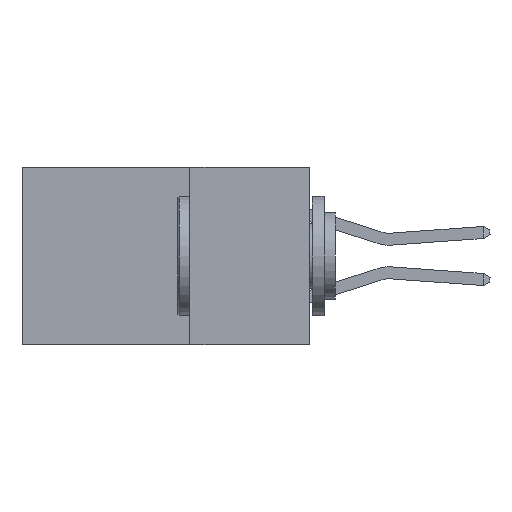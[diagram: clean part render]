
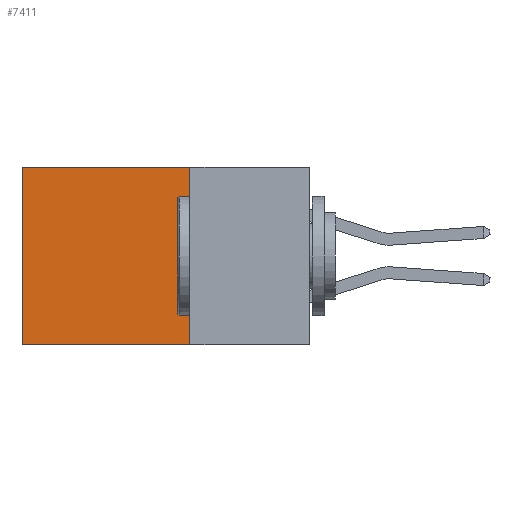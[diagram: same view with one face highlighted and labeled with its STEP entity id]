
A CAD part, left-side view. The second image highlights one B-rep face of the part: STEP entity #7411.
In plain terms, the highlighted planar face has unit normal (-1, 0, 0).
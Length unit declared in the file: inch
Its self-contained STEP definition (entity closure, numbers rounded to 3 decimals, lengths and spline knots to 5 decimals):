
#46 = CARTESIAN_POINT ( 'NONE',  ( 0.298, 0.6, -0.37 ) ) ;
#125 = VECTOR ( 'NONE', #10347, 39.37008 ) ;
#994 = CARTESIAN_POINT ( 'NONE',  ( 0.298, 0.25, 0. ) ) ;
#2013 = DIRECTION ( 'NONE',  ( 0., 1., 0. ) ) ;
#2755 = ORIENTED_EDGE ( 'NONE', *, *, #14834, .T. ) ;
#2896 = DIRECTION ( 'NONE',  ( 1., 0., 0. ) ) ;
#3699 = CARTESIAN_POINT ( 'NONE',  ( 0.298, 0.25, 0. ) ) ;
#4973 = ORIENTED_EDGE ( 'NONE', *, *, #9834, .F. ) ;
#5698 = VECTOR ( 'NONE', #7723, 39.37008 ) ;
#7411 = ADVANCED_FACE ( 'NONE', ( #11401 ), #12450, .F. ) ;
#7413 = ORIENTED_EDGE ( 'NONE', *, *, #21066, .T. ) ;
#7723 = DIRECTION ( 'NONE',  ( 0., 0., -1. ) ) ;
#9039 = EDGE_LOOP ( 'NONE', ( #2755, #11001, #4973, #7413 ) ) ;
#9103 = CARTESIAN_POINT ( 'NONE',  ( 0.298, 0.25, -0.37 ) ) ;
#9834 = EDGE_CURVE ( 'NONE', #15513, #27654, #18242, .T. ) ;
#10347 = DIRECTION ( 'NONE',  ( 0., 1., 0. ) ) ;
#11001 = ORIENTED_EDGE ( 'NONE', *, *, #12710, .F. ) ;
#11401 = FACE_OUTER_BOUND ( 'NONE', #9039, .T. ) ;
#12450 = PLANE ( 'NONE',  #20560 ) ;
#12710 = EDGE_CURVE ( 'NONE', #27654, #29159, #29627, .T. ) ;
#13726 = VERTEX_POINT ( 'NONE', #20423 ) ;
#14834 = EDGE_CURVE ( 'NONE', #13726, #29159, #23051, .T. ) ;
#15513 = VERTEX_POINT ( 'NONE', #3699 ) ;
#16161 = DIRECTION ( 'NONE',  ( 0., 0., -1. ) ) ;
#16728 = VECTOR ( 'NONE', #16161, 39.37008 ) ;
#18242 = LINE ( 'NONE', #21775, #5698 ) ;
#18309 = CARTESIAN_POINT ( 'NONE',  ( 0.298, 0.6, 0. ) ) ;
#19152 = CARTESIAN_POINT ( 'NONE',  ( 0.298, 0.25, 0. ) ) ;
#19452 = DIRECTION ( 'NONE',  ( 0., 0., -1. ) ) ;
#20139 = LINE ( 'NONE', #994, #125 ) ;
#20423 = CARTESIAN_POINT ( 'NONE',  ( 0.298, 0.6, 0. ) ) ;
#20560 = AXIS2_PLACEMENT_3D ( 'NONE', #19152, #2896, #19452 ) ;
#20646 = CARTESIAN_POINT ( 'NONE',  ( 0.298, 0.25, -0.37 ) ) ;
#21066 = EDGE_CURVE ( 'NONE', #15513, #13726, #20139, .T. ) ;
#21775 = CARTESIAN_POINT ( 'NONE',  ( 0.298, 0.25, 0. ) ) ;
#23051 = LINE ( 'NONE', #18309, #16728 ) ;
#23273 = VECTOR ( 'NONE', #2013, 39.37008 ) ;
#27654 = VERTEX_POINT ( 'NONE', #20646 ) ;
#29159 = VERTEX_POINT ( 'NONE', #46 ) ;
#29627 = LINE ( 'NONE', #9103, #23273 ) ;
